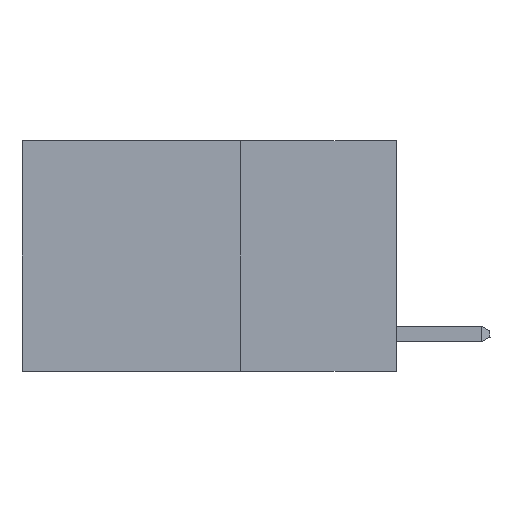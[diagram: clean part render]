
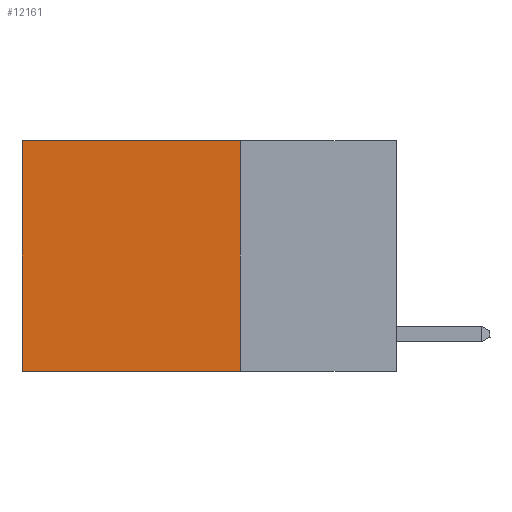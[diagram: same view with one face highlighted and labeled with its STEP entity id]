
A CAD part, left-side view. The second image highlights one B-rep face of the part: STEP entity #12161.
In plain terms, the highlighted planar face has unit normal (-1, 0, 0).
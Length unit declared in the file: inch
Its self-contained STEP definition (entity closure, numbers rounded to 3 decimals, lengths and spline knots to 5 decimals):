
#935 = VERTEX_POINT ( 'NONE', #14324 ) ;
#1076 = CARTESIAN_POINT ( 'NONE',  ( 0.2625, 0.25, -0.37 ) ) ;
#1093 = DIRECTION ( 'NONE',  ( 0., 1., 0. ) ) ;
#1391 = DIRECTION ( 'NONE',  ( 0., 0., -1. ) ) ;
#2591 = CARTESIAN_POINT ( 'NONE',  ( 0.2625, 0.25, 0. ) ) ;
#3643 = AXIS2_PLACEMENT_3D ( 'NONE', #12719, #13982, #6388 ) ;
#3948 = VERTEX_POINT ( 'NONE', #11655 ) ;
#4042 = CARTESIAN_POINT ( 'NONE',  ( 0.2625, 0.25, -0.37 ) ) ;
#4492 = ORIENTED_EDGE ( 'NONE', *, *, #6632, .T. ) ;
#4633 = VECTOR ( 'NONE', #12694, 39.37008 ) ;
#5325 = DIRECTION ( 'NONE',  ( 0., 1., 0. ) ) ;
#6017 = ORIENTED_EDGE ( 'NONE', *, *, #14036, .F. ) ;
#6388 = DIRECTION ( 'NONE',  ( 0., 0., -1. ) ) ;
#6632 = EDGE_CURVE ( 'NONE', #12182, #935, #11430, .T. ) ;
#6658 = EDGE_CURVE ( 'NONE', #12182, #7254, #14779, .T. ) ;
#7254 = VERTEX_POINT ( 'NONE', #1076 ) ;
#7601 = CARTESIAN_POINT ( 'NONE',  ( 0.2625, 0.25, 0. ) ) ;
#7826 = CARTESIAN_POINT ( 'NONE',  ( 0.2625, 0.6, 0. ) ) ;
#8064 = VECTOR ( 'NONE', #1093, 39.37008 ) ;
#8213 = VECTOR ( 'NONE', #1391, 39.37008 ) ;
#8232 = EDGE_CURVE ( 'NONE', #935, #3948, #11169, .T. ) ;
#8903 = LINE ( 'NONE', #4042, #15233 ) ;
#10772 = EDGE_LOOP ( 'NONE', ( #16600, #6017, #15886, #4492 ) ) ;
#11169 = LINE ( 'NONE', #7826, #8213 ) ;
#11430 = LINE ( 'NONE', #16375, #8064 ) ;
#11454 = PLANE ( 'NONE',  #3643 ) ;
#11655 = CARTESIAN_POINT ( 'NONE',  ( 0.2625, 0.6, -0.37 ) ) ;
#12161 = ADVANCED_FACE ( 'NONE', ( #15585 ), #11454, .F. ) ;
#12182 = VERTEX_POINT ( 'NONE', #2591 ) ;
#12694 = DIRECTION ( 'NONE',  ( 0., 0., -1. ) ) ;
#12719 = CARTESIAN_POINT ( 'NONE',  ( 0.2625, 0.25, 0. ) ) ;
#13982 = DIRECTION ( 'NONE',  ( 1., 0., 0. ) ) ;
#14036 = EDGE_CURVE ( 'NONE', #7254, #3948, #8903, .T. ) ;
#14324 = CARTESIAN_POINT ( 'NONE',  ( 0.2625, 0.6, 0. ) ) ;
#14779 = LINE ( 'NONE', #7601, #4633 ) ;
#15233 = VECTOR ( 'NONE', #5325, 39.37008 ) ;
#15585 = FACE_OUTER_BOUND ( 'NONE', #10772, .T. ) ;
#15886 = ORIENTED_EDGE ( 'NONE', *, *, #6658, .F. ) ;
#16375 = CARTESIAN_POINT ( 'NONE',  ( 0.2625, 0.25, 0. ) ) ;
#16600 = ORIENTED_EDGE ( 'NONE', *, *, #8232, .T. ) ;
